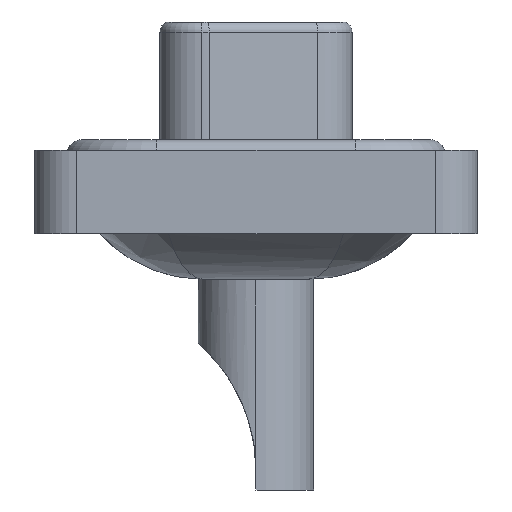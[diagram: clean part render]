
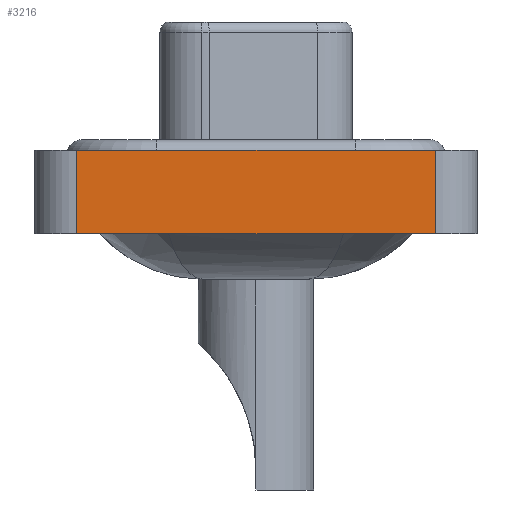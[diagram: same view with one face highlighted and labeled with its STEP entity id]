
A CAD part, left-side view. The second image highlights one B-rep face of the part: STEP entity #3216.
In plain terms, the highlighted planar face has unit normal (-1, 0, 0).
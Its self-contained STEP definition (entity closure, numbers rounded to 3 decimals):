
#222 = VECTOR ( 'NONE', #5893, 1000. ) ;
#266 = VERTEX_POINT ( 'NONE', #14553 ) ;
#509 = EDGE_LOOP ( 'NONE', ( #12070, #6658, #9208, #6737 ) ) ;
#865 = PLANE ( 'NONE',  #18049 ) ;
#1134 = FACE_OUTER_BOUND ( 'NONE', #509, .T. ) ;
#1325 = VERTEX_POINT ( 'NONE', #5454 ) ;
#2654 = LINE ( 'NONE', #14121, #10133 ) ;
#3188 = VERTEX_POINT ( 'NONE', #13369 ) ;
#3216 = ADVANCED_FACE ( 'NONE', ( #1134 ), #865, .T. ) ;
#3266 = CARTESIAN_POINT ( 'NONE',  ( -7.25, -8.55, -3.6 ) ) ;
#4459 = EDGE_CURVE ( 'NONE', #3188, #1325, #2654, .T. ) ;
#5454 = CARTESIAN_POINT ( 'NONE',  ( -7.25, -8.55, 0.4 ) ) ;
#5481 = VERTEX_POINT ( 'NONE', #13520 ) ;
#5893 = DIRECTION ( 'NONE',  ( 0., 0., 1. ) ) ;
#6658 = ORIENTED_EDGE ( 'NONE', *, *, #8056, .F. ) ;
#6737 = ORIENTED_EDGE ( 'NONE', *, *, #7362, .T. ) ;
#7362 = EDGE_CURVE ( 'NONE', #266, #3188, #11683, .T. ) ;
#8056 = EDGE_CURVE ( 'NONE', #5481, #1325, #11349, .T. ) ;
#8630 = LINE ( 'NONE', #14270, #222 ) ;
#9208 = ORIENTED_EDGE ( 'NONE', *, *, #16947, .F. ) ;
#9697 = DIRECTION ( 'NONE',  ( 0., 0., 1. ) ) ;
#9797 = DIRECTION ( 'NONE',  ( 0., -1., 0. ) ) ;
#10133 = VECTOR ( 'NONE', #9697, 1000. ) ;
#10911 = DIRECTION ( 'NONE',  ( 0., 0., 1. ) ) ;
#11349 = LINE ( 'NONE', #13970, #12840 ) ;
#11683 = LINE ( 'NONE', #3266, #12242 ) ;
#12070 = ORIENTED_EDGE ( 'NONE', *, *, #4459, .T. ) ;
#12242 = VECTOR ( 'NONE', #17138, 1000. ) ;
#12840 = VECTOR ( 'NONE', #9797, 1000. ) ;
#13369 = CARTESIAN_POINT ( 'NONE',  ( -7.25, -8.55, -3.6 ) ) ;
#13520 = CARTESIAN_POINT ( 'NONE',  ( -7.25, 8.55, 0.4 ) ) ;
#13970 = CARTESIAN_POINT ( 'NONE',  ( -7.25, -8.55, 0.4 ) ) ;
#14121 = CARTESIAN_POINT ( 'NONE',  ( -7.25, -8.55, -3.6 ) ) ;
#14270 = CARTESIAN_POINT ( 'NONE',  ( -7.25, 8.55, -3.6 ) ) ;
#14553 = CARTESIAN_POINT ( 'NONE',  ( -7.25, 8.55, -3.6 ) ) ;
#16947 = EDGE_CURVE ( 'NONE', #266, #5481, #8630, .T. ) ;
#17138 = DIRECTION ( 'NONE',  ( 0., -1., 0. ) ) ;
#17850 = CARTESIAN_POINT ( 'NONE',  ( -7.25, -8.55, -3.6 ) ) ;
#17926 = DIRECTION ( 'NONE',  ( -1., 0., 0. ) ) ;
#18049 = AXIS2_PLACEMENT_3D ( 'NONE', #17850, #17926, #10911 ) ;
